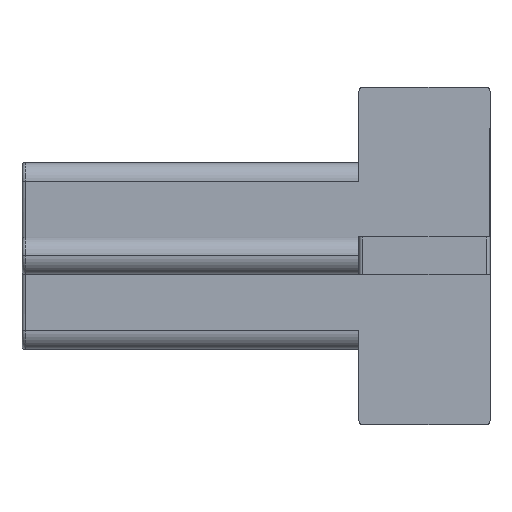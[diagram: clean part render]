
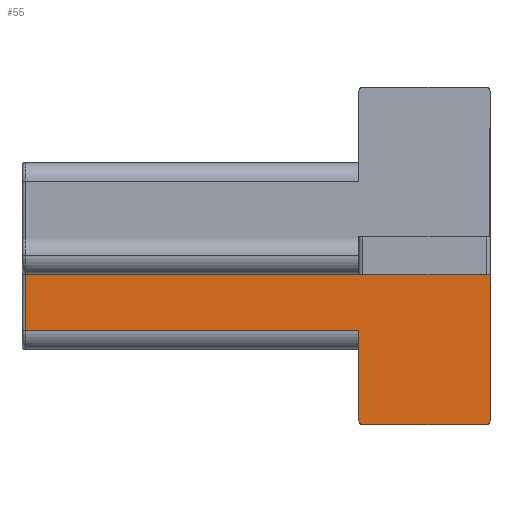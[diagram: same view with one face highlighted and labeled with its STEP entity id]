
A CAD part, top view. The second image highlights one B-rep face of the part: STEP entity #55.
In plain terms, the highlighted planar face has unit normal (0, 0, 1).
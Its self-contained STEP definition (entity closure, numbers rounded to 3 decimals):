
#28 = LINE ( 'NONE', #1109, #46 ) ;
#46 = VECTOR ( 'NONE', #1088, 1000. ) ;
#55 = ADVANCED_FACE ( 'NONE', ( #462 ), #99, .F. ) ;
#94 = CARTESIAN_POINT ( 'NONE',  ( 9.5, 2.5, 0.5 ) ) ;
#99 = PLANE ( 'NONE',  #332 ) ;
#130 = DIRECTION ( 'NONE',  ( 0., 1., 0. ) ) ;
#131 = DIRECTION ( 'NONE',  ( 0., 0., -1. ) ) ;
#172 = EDGE_CURVE ( 'NONE', #1370, #1371, #28, .T. ) ;
#260 = VECTOR ( 'NONE', #924, 1000. ) ;
#261 = CIRCLE ( 'NONE', #1009, 0.1 ) ;
#263 = LINE ( 'NONE', #933, #260 ) ;
#286 = VECTOR ( 'NONE', #602, 1000. ) ;
#288 = VECTOR ( 'NONE', #625, 1000. ) ;
#289 = LINE ( 'NONE', #603, #286 ) ;
#291 = LINE ( 'NONE', #626, #288 ) ;
#292 = VECTOR ( 'NONE', #613, 1000. ) ;
#293 = CIRCLE ( 'NONE', #990, 0.1 ) ;
#294 = VECTOR ( 'NONE', #615, 1000. ) ;
#295 = LINE ( 'NONE', #614, #292 ) ;
#297 = LINE ( 'NONE', #617, #294 ) ;
#332 = AXIS2_PLACEMENT_3D ( 'NONE', #94, #131, #130 ) ;
#355 = EDGE_CURVE ( 'NONE', #1355, #1370, #297, .T. ) ;
#356 = EDGE_CURVE ( 'NONE', #1321, #1371, #295, .T. ) ;
#357 = EDGE_CURVE ( 'NONE', #1321, #1342, #293, .T. ) ;
#358 = EDGE_CURVE ( 'NONE', #1289, #1346, #291, .T. ) ;
#359 = EDGE_CURVE ( 'NONE', #1355, #1289, #289, .T. ) ;
#396 = EDGE_CURVE ( 'NONE', #1396, #1342, #263, .T. ) ;
#397 = EDGE_CURVE ( 'NONE', #1396, #1346, #261, .T. ) ;
#462 = FACE_OUTER_BOUND ( 'NONE', #1409, .T. ) ;
#475 = ORIENTED_EDGE ( 'NONE', *, *, #358, .F. ) ;
#477 = ORIENTED_EDGE ( 'NONE', *, *, #359, .F. ) ;
#478 = ORIENTED_EDGE ( 'NONE', *, *, #396, .F. ) ;
#479 = ORIENTED_EDGE ( 'NONE', *, *, #397, .T. ) ;
#480 = ORIENTED_EDGE ( 'NONE', *, *, #356, .F. ) ;
#481 = ORIENTED_EDGE ( 'NONE', *, *, #357, .T. ) ;
#482 = ORIENTED_EDGE ( 'NONE', *, *, #355, .T. ) ;
#483 = ORIENTED_EDGE ( 'NONE', *, *, #172, .T. ) ;
#602 = DIRECTION ( 'NONE',  ( 1., 0., 0. ) ) ;
#603 = CARTESIAN_POINT ( 'NONE',  ( 9.5, -0.5, 0.5 ) ) ;
#604 = DIRECTION ( 'NONE',  ( 0., 1., 0. ) ) ;
#605 = DIRECTION ( 'NONE',  ( 0., 0., 1. ) ) ;
#607 = CARTESIAN_POINT ( 'NONE',  ( 6.1, -4.4, 0.5 ) ) ;
#613 = DIRECTION ( 'NONE',  ( 0., 1., 0. ) ) ;
#614 = CARTESIAN_POINT ( 'NONE',  ( 6., -4.5, 0.5 ) ) ;
#615 = DIRECTION ( 'NONE',  ( 0., -1., 0. ) ) ;
#617 = CARTESIAN_POINT ( 'NONE',  ( -2.9, -2.5, 0.5 ) ) ;
#625 = DIRECTION ( 'NONE',  ( 0., -1., 0. ) ) ;
#626 = CARTESIAN_POINT ( 'NONE',  ( 9.5, 2.5, 0.5 ) ) ;
#875 = CARTESIAN_POINT ( 'NONE',  ( 6.1, -4.5, 0.5 ) ) ;
#882 = CARTESIAN_POINT ( 'NONE',  ( 9.5, -4.4, 0.5 ) ) ;
#888 = CARTESIAN_POINT ( 'NONE',  ( 6., -4.4, 0.5 ) ) ;
#910 = CARTESIAN_POINT ( 'NONE',  ( 9.5, -0.5, 0.5 ) ) ;
#911 = DIRECTION ( 'NONE',  ( 0., 1., 0. ) ) ;
#913 = DIRECTION ( 'NONE',  ( 0., 0., 1. ) ) ;
#917 = CARTESIAN_POINT ( 'NONE',  ( 9.4, -4.4, 0.5 ) ) ;
#924 = DIRECTION ( 'NONE',  ( -1., 0., 0. ) ) ;
#933 = CARTESIAN_POINT ( 'NONE',  ( 9.5, -4.5, 0.5 ) ) ;
#938 = CARTESIAN_POINT ( 'NONE',  ( 9.4, -4.5, 0.5 ) ) ;
#956 = CARTESIAN_POINT ( 'NONE',  ( 6., -2., 0.5 ) ) ;
#957 = CARTESIAN_POINT ( 'NONE',  ( -2.9, -2., 0.5 ) ) ;
#975 = CARTESIAN_POINT ( 'NONE',  ( -2.9, -0.5, 0.5 ) ) ;
#990 = AXIS2_PLACEMENT_3D ( 'NONE', #607, #605, #604 ) ;
#1009 = AXIS2_PLACEMENT_3D ( 'NONE', #917, #913, #911 ) ;
#1088 = DIRECTION ( 'NONE',  ( 1., 0., 0. ) ) ;
#1109 = CARTESIAN_POINT ( 'NONE',  ( 9.5, -2., 0.5 ) ) ;
#1289 = VERTEX_POINT ( 'NONE', #910 ) ;
#1321 = VERTEX_POINT ( 'NONE', #888 ) ;
#1342 = VERTEX_POINT ( 'NONE', #875 ) ;
#1346 = VERTEX_POINT ( 'NONE', #882 ) ;
#1355 = VERTEX_POINT ( 'NONE', #975 ) ;
#1370 = VERTEX_POINT ( 'NONE', #957 ) ;
#1371 = VERTEX_POINT ( 'NONE', #956 ) ;
#1396 = VERTEX_POINT ( 'NONE', #938 ) ;
#1409 = EDGE_LOOP ( 'NONE', ( #482, #483, #480, #481, #478, #479, #475, #477 ) ) ;
